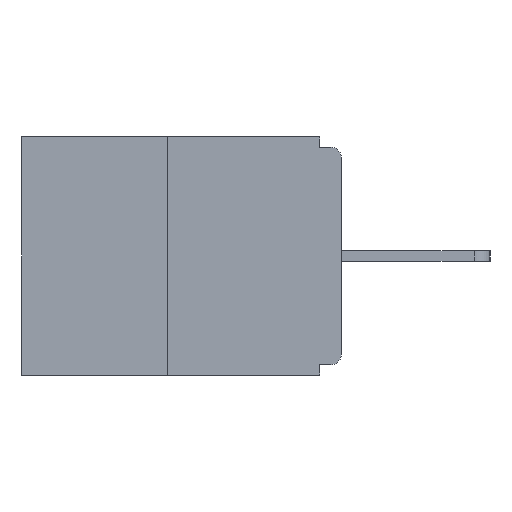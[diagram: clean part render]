
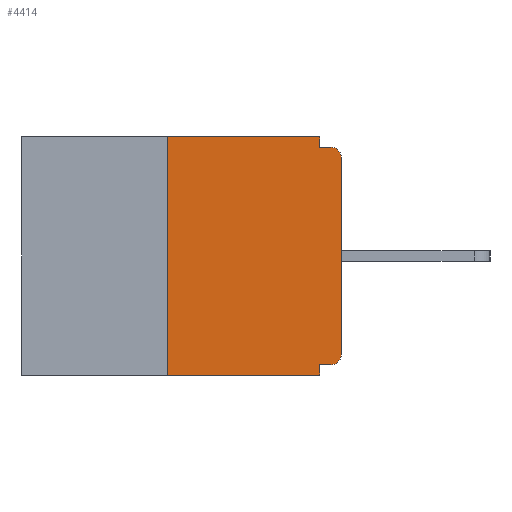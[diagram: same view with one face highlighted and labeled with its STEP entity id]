
A CAD part, left-side view. The second image highlights one B-rep face of the part: STEP entity #4414.
In plain terms, the highlighted planar face has unit normal (-1, 0, 0).
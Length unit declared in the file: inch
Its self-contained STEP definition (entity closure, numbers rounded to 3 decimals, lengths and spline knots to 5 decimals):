
#264 = CARTESIAN_POINT ( 'NONE',  ( 0., 0., -0.328 ) ) ;
#704 = ORIENTED_EDGE ( 'NONE', *, *, #14211, .F. ) ;
#964 = DIRECTION ( 'NONE',  ( 0., 0., -1. ) ) ;
#969 = EDGE_CURVE ( 'NONE', #7799, #10455, #1196, .T. ) ;
#1030 = VECTOR ( 'NONE', #17217, 39.37008 ) ;
#1195 = CARTESIAN_POINT ( 'NONE',  ( 0., 0.031, -0.343 ) ) ;
#1196 = LINE ( 'NONE', #8540, #4717 ) ;
#1311 = CIRCLE ( 'NONE', #17251, 0.015 ) ;
#1319 = VECTOR ( 'NONE', #7628, 39.37008 ) ;
#1325 = DIRECTION ( 'NONE',  ( 1., 0., 0. ) ) ;
#1770 = CARTESIAN_POINT ( 'NONE',  ( 0., 0.46, 0. ) ) ;
#1827 = VERTEX_POINT ( 'NONE', #10592 ) ;
#1926 = DIRECTION ( 'NONE',  ( 0., 0., 1. ) ) ;
#2007 = LINE ( 'NONE', #3142, #1319 ) ;
#2736 = EDGE_CURVE ( 'NONE', #4288, #11905, #1311, .T. ) ;
#3090 = EDGE_LOOP ( 'NONE', ( #5250, #6259, #4162, #704, #18135, #8964, #10609, #11459, #8467, #15486 ) ) ;
#3098 = CARTESIAN_POINT ( 'NONE',  ( 0., 0.25, 0. ) ) ;
#3109 = VERTEX_POINT ( 'NONE', #12178 ) ;
#3142 = CARTESIAN_POINT ( 'NONE',  ( 0., 0., -0.015 ) ) ;
#3186 = EDGE_CURVE ( 'NONE', #14024, #4288, #10694, .T. ) ;
#3230 = VECTOR ( 'NONE', #4680, 39.37008 ) ;
#3545 = VECTOR ( 'NONE', #6916, 39.37008 ) ;
#4162 = ORIENTED_EDGE ( 'NONE', *, *, #17646, .T. ) ;
#4288 = VERTEX_POINT ( 'NONE', #12156 ) ;
#4414 = ADVANCED_FACE ( 'NONE', ( #14223 ), #8317, .F. ) ;
#4563 = EDGE_CURVE ( 'NONE', #17799, #1827, #5741, .T. ) ;
#4659 = CARTESIAN_POINT ( 'NONE',  ( 0., 0.015, -0.015 ) ) ;
#4680 = DIRECTION ( 'NONE',  ( 0., 0., 1. ) ) ;
#4717 = VECTOR ( 'NONE', #8453, 39.37008 ) ;
#4965 = AXIS2_PLACEMENT_3D ( 'NONE', #12681, #9757, #15397 ) ;
#5248 = DIRECTION ( 'NONE',  ( -1., 0., 0. ) ) ;
#5250 = ORIENTED_EDGE ( 'NONE', *, *, #11812, .F. ) ;
#5741 = LINE ( 'NONE', #264, #10498 ) ;
#5820 = DIRECTION ( 'NONE',  ( 0., 1., 0. ) ) ;
#6131 = CIRCLE ( 'NONE', #4965, 0.015 ) ;
#6259 = ORIENTED_EDGE ( 'NONE', *, *, #15127, .F. ) ;
#6353 = CARTESIAN_POINT ( 'NONE',  ( 0., 0., -0.313 ) ) ;
#6355 = LINE ( 'NONE', #3098, #3230 ) ;
#6378 = DIRECTION ( 'NONE',  ( 0., 0., -1. ) ) ;
#6669 = CARTESIAN_POINT ( 'NONE',  ( 0., 0.031, 0. ) ) ;
#6916 = DIRECTION ( 'NONE',  ( 0., 0., -1. ) ) ;
#7194 = LINE ( 'NONE', #1195, #3545 ) ;
#7485 = CARTESIAN_POINT ( 'NONE',  ( 0., 0.015, -0.328 ) ) ;
#7628 = DIRECTION ( 'NONE',  ( 0., -1., 0. ) ) ;
#7799 = VERTEX_POINT ( 'NONE', #6669 ) ;
#8317 = PLANE ( 'NONE',  #12289 ) ;
#8453 = DIRECTION ( 'NONE',  ( 0., 0., -1. ) ) ;
#8467 = ORIENTED_EDGE ( 'NONE', *, *, #17172, .F. ) ;
#8540 = CARTESIAN_POINT ( 'NONE',  ( 0., 0.031, 0. ) ) ;
#8554 = LINE ( 'NONE', #12877, #1030 ) ;
#8964 = ORIENTED_EDGE ( 'NONE', *, *, #10726, .T. ) ;
#9757 = DIRECTION ( 'NONE',  ( -1., 0., 0. ) ) ;
#9812 = CARTESIAN_POINT ( 'NONE',  ( 0., 0.46, 0. ) ) ;
#10455 = VERTEX_POINT ( 'NONE', #13728 ) ;
#10495 = VECTOR ( 'NONE', #13248, 39.37008 ) ;
#10498 = VECTOR ( 'NONE', #5820, 39.37008 ) ;
#10592 = CARTESIAN_POINT ( 'NONE',  ( 0., 0.031, -0.328 ) ) ;
#10609 = ORIENTED_EDGE ( 'NONE', *, *, #3186, .T. ) ;
#10694 = LINE ( 'NONE', #10886, #16970 ) ;
#10726 = EDGE_CURVE ( 'NONE', #17799, #14024, #6131, .T. ) ;
#10886 = CARTESIAN_POINT ( 'NONE',  ( 0., 0., 0. ) ) ;
#11165 = VERTEX_POINT ( 'NONE', #14289 ) ;
#11253 = VERTEX_POINT ( 'NONE', #18154 ) ;
#11459 = ORIENTED_EDGE ( 'NONE', *, *, #2736, .T. ) ;
#11812 = EDGE_CURVE ( 'NONE', #11253, #7799, #17584, .T. ) ;
#11905 = VERTEX_POINT ( 'NONE', #4659 ) ;
#12156 = CARTESIAN_POINT ( 'NONE',  ( 0., 0., -0.03 ) ) ;
#12178 = CARTESIAN_POINT ( 'NONE',  ( 0., 0.031, -0.343 ) ) ;
#12289 = AXIS2_PLACEMENT_3D ( 'NONE', #9812, #1325, #964 ) ;
#12681 = CARTESIAN_POINT ( 'NONE',  ( 0., 0.015, -0.313 ) ) ;
#12877 = CARTESIAN_POINT ( 'NONE',  ( 0., 0.46, -0.343 ) ) ;
#13248 = DIRECTION ( 'NONE',  ( 0., -1., 0. ) ) ;
#13728 = CARTESIAN_POINT ( 'NONE',  ( 0., 0.031, -0.015 ) ) ;
#14024 = VERTEX_POINT ( 'NONE', #6353 ) ;
#14211 = EDGE_CURVE ( 'NONE', #1827, #3109, #7194, .T. ) ;
#14223 = FACE_OUTER_BOUND ( 'NONE', #3090, .T. ) ;
#14289 = CARTESIAN_POINT ( 'NONE',  ( 0., 0.25, -0.343 ) ) ;
#15127 = EDGE_CURVE ( 'NONE', #11165, #11253, #6355, .T. ) ;
#15397 = DIRECTION ( 'NONE',  ( 0., 0., -1. ) ) ;
#15486 = ORIENTED_EDGE ( 'NONE', *, *, #969, .F. ) ;
#16970 = VECTOR ( 'NONE', #1926, 39.37008 ) ;
#17172 = EDGE_CURVE ( 'NONE', #10455, #11905, #2007, .T. ) ;
#17217 = DIRECTION ( 'NONE',  ( 0., -1., 0. ) ) ;
#17251 = AXIS2_PLACEMENT_3D ( 'NONE', #18188, #5248, #6378 ) ;
#17584 = LINE ( 'NONE', #1770, #10495 ) ;
#17646 = EDGE_CURVE ( 'NONE', #11165, #3109, #8554, .T. ) ;
#17799 = VERTEX_POINT ( 'NONE', #7485 ) ;
#18135 = ORIENTED_EDGE ( 'NONE', *, *, #4563, .F. ) ;
#18154 = CARTESIAN_POINT ( 'NONE',  ( 0., 0.25, 0. ) ) ;
#18188 = CARTESIAN_POINT ( 'NONE',  ( 0., 0.015, -0.03 ) ) ;
